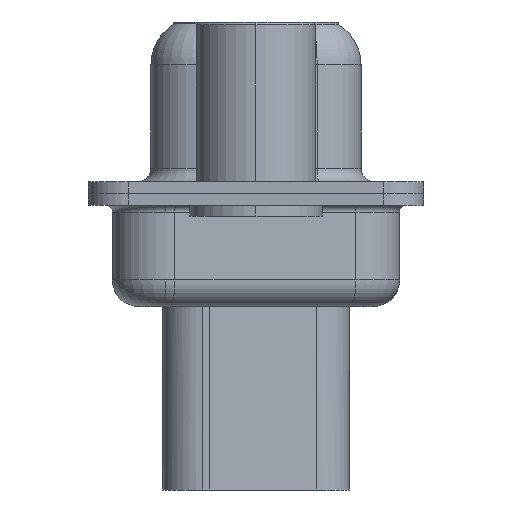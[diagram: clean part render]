
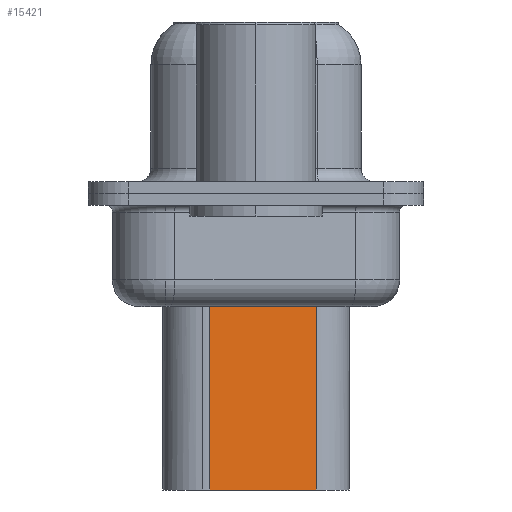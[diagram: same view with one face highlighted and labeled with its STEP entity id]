
A CAD part, left-side view. The second image highlights one B-rep face of the part: STEP entity #15421.
In plain terms, the highlighted planar face has unit normal (-0.985, -0.174, 0).
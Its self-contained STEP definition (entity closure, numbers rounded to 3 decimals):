
#889 = VERTEX_POINT ( 'NONE', #6734 ) ;
#2078 = CARTESIAN_POINT ( 'NONE',  ( 4.524, 1.74, -3.1 ) ) ;
#2349 = VECTOR ( 'NONE', #6000, 1000. ) ;
#2465 = ORIENTED_EDGE ( 'NONE', *, *, #8979, .F. ) ;
#3385 = CARTESIAN_POINT ( 'NONE',  ( 5.229, -2.26, -3.975 ) ) ;
#3545 = VECTOR ( 'NONE', #14385, 1000. ) ;
#3748 = ORIENTED_EDGE ( 'NONE', *, *, #13972, .T. ) ;
#4374 = EDGE_CURVE ( 'NONE', #8526, #889, #21456, .T. ) ;
#4772 = EDGE_LOOP ( 'NONE', ( #13891, #3748, #18854, #2465 ) ) ;
#5279 = LINE ( 'NONE', #23535, #21001 ) ;
#6000 = DIRECTION ( 'NONE',  ( 0., 0., -1. ) ) ;
#6485 = AXIS2_PLACEMENT_3D ( 'NONE', #19148, #10330, #8667 ) ;
#6734 = CARTESIAN_POINT ( 'NONE',  ( 5.229, -2.26, -11.15 ) ) ;
#8435 = FACE_OUTER_BOUND ( 'NONE', #4772, .T. ) ;
#8526 = VERTEX_POINT ( 'NONE', #3385 ) ;
#8667 = DIRECTION ( 'NONE',  ( 0.174, -0.985, 0. ) ) ;
#8672 = CARTESIAN_POINT ( 'NONE',  ( 5.229, -2.26, -3.1 ) ) ;
#8673 = EDGE_CURVE ( 'NONE', #19119, #12329, #18733, .T. ) ;
#8979 = EDGE_CURVE ( 'NONE', #889, #12329, #5279, .T. ) ;
#8985 = CARTESIAN_POINT ( 'NONE',  ( 4.524, 1.74, -11.15 ) ) ;
#10330 = DIRECTION ( 'NONE',  ( -0.985, -0.174, 0. ) ) ;
#10614 = DIRECTION ( 'NONE',  ( -0.174, 0.985, 0. ) ) ;
#11833 = CARTESIAN_POINT ( 'NONE',  ( 4.353, 2.709, -3.975 ) ) ;
#12329 = VERTEX_POINT ( 'NONE', #8985 ) ;
#13891 = ORIENTED_EDGE ( 'NONE', *, *, #4374, .F. ) ;
#13972 = EDGE_CURVE ( 'NONE', #8526, #19119, #22590, .T. ) ;
#14385 = DIRECTION ( 'NONE',  ( 0., 0., -1. ) ) ;
#15393 = DIRECTION ( 'NONE',  ( -0.174, 0.985, 0. ) ) ;
#15421 = ADVANCED_FACE ( 'NONE', ( #8435 ), #15688, .T. ) ;
#15688 = PLANE ( 'NONE',  #6485 ) ;
#15718 = VECTOR ( 'NONE', #15393, 1000. ) ;
#17164 = CARTESIAN_POINT ( 'NONE',  ( 4.524, 1.74, -3.975 ) ) ;
#18733 = LINE ( 'NONE', #2078, #2349 ) ;
#18854 = ORIENTED_EDGE ( 'NONE', *, *, #8673, .T. ) ;
#19119 = VERTEX_POINT ( 'NONE', #17164 ) ;
#19148 = CARTESIAN_POINT ( 'NONE',  ( 4.524, 1.74, -3.1 ) ) ;
#21001 = VECTOR ( 'NONE', #10614, 1000. ) ;
#21456 = LINE ( 'NONE', #8672, #3545 ) ;
#22590 = LINE ( 'NONE', #11833, #15718 ) ;
#23535 = CARTESIAN_POINT ( 'NONE',  ( 4.524, 1.74, -11.15 ) ) ;
